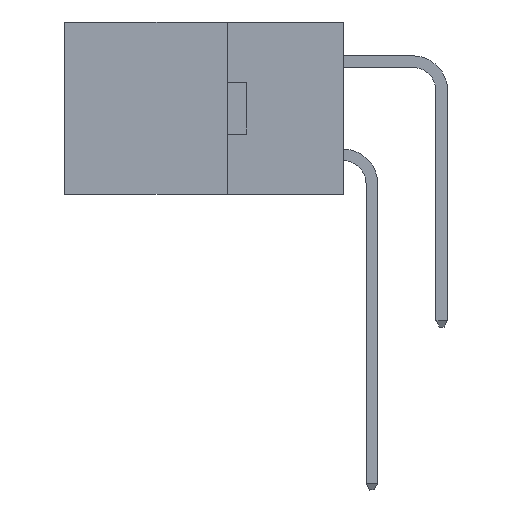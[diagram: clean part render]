
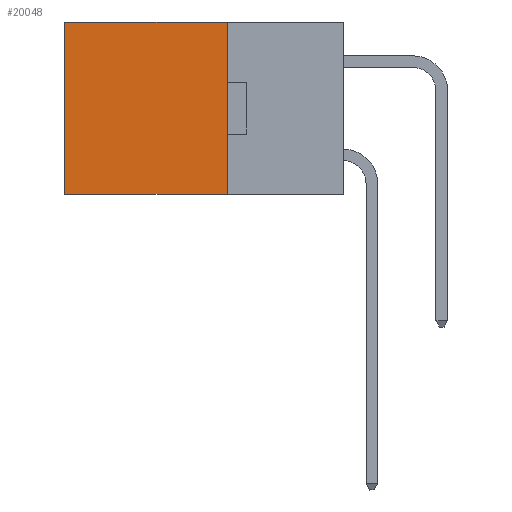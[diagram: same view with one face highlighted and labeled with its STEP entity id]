
A CAD part, left-side view. The second image highlights one B-rep face of the part: STEP entity #20048.
In plain terms, the highlighted planar face has unit normal (-1, 0, 0).
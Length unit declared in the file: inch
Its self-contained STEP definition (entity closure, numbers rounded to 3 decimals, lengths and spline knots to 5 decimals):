
#144 = CARTESIAN_POINT ( 'NONE',  ( 0.2615, 0.25, 0. ) ) ;
#1635 = LINE ( 'NONE', #10618, #23479 ) ;
#5021 = EDGE_LOOP ( 'NONE', ( #13365, #19171, #8102, #25266 ) ) ;
#5660 = AXIS2_PLACEMENT_3D ( 'NONE', #22815, #8899, #25127 ) ;
#6019 = VERTEX_POINT ( 'NONE', #26162 ) ;
#7198 = DIRECTION ( 'NONE',  ( 0., 1., 0. ) ) ;
#7280 = EDGE_CURVE ( 'NONE', #8684, #6019, #23513, .T. ) ;
#7994 = CARTESIAN_POINT ( 'NONE',  ( 0.2615, 0.25, 0. ) ) ;
#8102 = ORIENTED_EDGE ( 'NONE', *, *, #20582, .F. ) ;
#8599 = VERTEX_POINT ( 'NONE', #7994 ) ;
#8684 = VERTEX_POINT ( 'NONE', #29042 ) ;
#8899 = DIRECTION ( 'NONE',  ( 1., 0., 0. ) ) ;
#10126 = CARTESIAN_POINT ( 'NONE',  ( 0.2615, 0.25, -0.37 ) ) ;
#10248 = VECTOR ( 'NONE', #11481, 39.37008 ) ;
#10618 = CARTESIAN_POINT ( 'NONE',  ( 0.2615, 0.25, -0.37 ) ) ;
#11481 = DIRECTION ( 'NONE',  ( 0., 0., -1. ) ) ;
#13159 = VERTEX_POINT ( 'NONE', #24788 ) ;
#13365 = ORIENTED_EDGE ( 'NONE', *, *, #16837, .T. ) ;
#16117 = VECTOR ( 'NONE', #7198, 39.37008 ) ;
#16837 = EDGE_CURVE ( 'NONE', #13159, #6019, #28682, .T. ) ;
#17382 = VECTOR ( 'NONE', #19476, 39.37008 ) ;
#18195 = PLANE ( 'NONE',  #5660 ) ;
#19171 = ORIENTED_EDGE ( 'NONE', *, *, #7280, .F. ) ;
#19476 = DIRECTION ( 'NONE',  ( 0., 1., 0. ) ) ;
#19532 = FACE_OUTER_BOUND ( 'NONE', #5021, .T. ) ;
#20048 = ADVANCED_FACE ( 'NONE', ( #19532 ), #18195, .F. ) ;
#20582 = EDGE_CURVE ( 'NONE', #8599, #8684, #1635, .T. ) ;
#22815 = CARTESIAN_POINT ( 'NONE',  ( 0.2615, 0.25, -0.37 ) ) ;
#23264 = EDGE_CURVE ( 'NONE', #8599, #13159, #28306, .T. ) ;
#23479 = VECTOR ( 'NONE', #24382, 39.37008 ) ;
#23513 = LINE ( 'NONE', #10126, #17382 ) ;
#24382 = DIRECTION ( 'NONE',  ( 0., 0., -1. ) ) ;
#24788 = CARTESIAN_POINT ( 'NONE',  ( 0.2615, 0.6, 0. ) ) ;
#25127 = DIRECTION ( 'NONE',  ( 0., 0., -1. ) ) ;
#25266 = ORIENTED_EDGE ( 'NONE', *, *, #23264, .T. ) ;
#26162 = CARTESIAN_POINT ( 'NONE',  ( 0.2615, 0.6, -0.37 ) ) ;
#27627 = CARTESIAN_POINT ( 'NONE',  ( 0.2615, 0.6, -0.37 ) ) ;
#28306 = LINE ( 'NONE', #144, #16117 ) ;
#28682 = LINE ( 'NONE', #27627, #10248 ) ;
#29042 = CARTESIAN_POINT ( 'NONE',  ( 0.2615, 0.25, -0.37 ) ) ;
